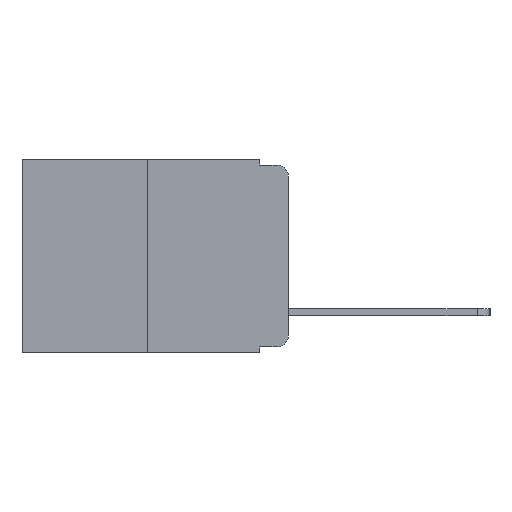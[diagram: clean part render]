
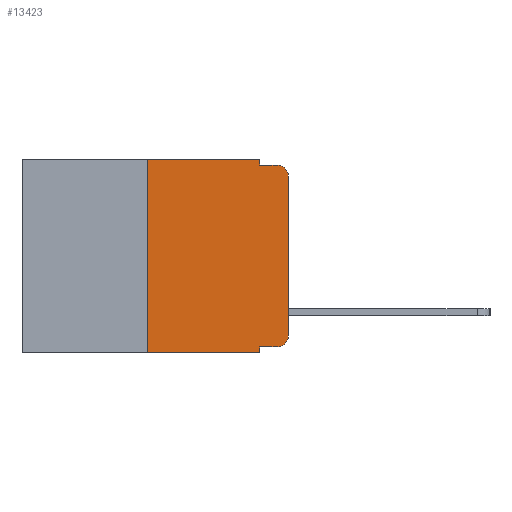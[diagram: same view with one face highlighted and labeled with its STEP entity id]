
A CAD part, left-side view. The second image highlights one B-rep face of the part: STEP entity #13423.
In plain terms, the highlighted planar face has unit normal (-1, 0, 0).
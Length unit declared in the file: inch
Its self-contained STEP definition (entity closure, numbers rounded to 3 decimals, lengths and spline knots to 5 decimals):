
#88 = AXIS2_PLACEMENT_3D ( 'NONE', #2605, #11744, #22862 ) ;
#1065 = CARTESIAN_POINT ( 'NONE',  ( 0., 0.051, 0. ) ) ;
#1620 = DIRECTION ( 'NONE',  ( 0., 0., 1. ) ) ;
#1627 = CARTESIAN_POINT ( 'NONE',  ( 0., 0.051, -0.01 ) ) ;
#1866 = EDGE_CURVE ( 'NONE', #9537, #21840, #20682, .T. ) ;
#1930 = VERTEX_POINT ( 'NONE', #1065 ) ;
#2000 = LINE ( 'NONE', #10922, #16400 ) ;
#2103 = LINE ( 'NONE', #11504, #17095 ) ;
#2592 = VECTOR ( 'NONE', #14992, 39.37008 ) ;
#2605 = CARTESIAN_POINT ( 'NONE',  ( 0., 0.02, -0.03 ) ) ;
#2713 = VERTEX_POINT ( 'NONE', #7784 ) ;
#3090 = LINE ( 'NONE', #24784, #12928 ) ;
#3095 = VECTOR ( 'NONE', #11310, 39.37008 ) ;
#3607 = VERTEX_POINT ( 'NONE', #5575 ) ;
#3814 = CARTESIAN_POINT ( 'NONE',  ( 0., 0.02, -0.333 ) ) ;
#4448 = CARTESIAN_POINT ( 'NONE',  ( 0., 0.051, 0. ) ) ;
#5096 = EDGE_CURVE ( 'NONE', #22543, #3607, #7813, .T. ) ;
#5575 = CARTESIAN_POINT ( 'NONE',  ( 0., 0.051, -0.343 ) ) ;
#5905 = ORIENTED_EDGE ( 'NONE', *, *, #12785, .T. ) ;
#6699 = EDGE_CURVE ( 'NONE', #22543, #2713, #17188, .T. ) ;
#6916 = CIRCLE ( 'NONE', #16382, 0.02 ) ;
#7174 = DIRECTION ( 'NONE',  ( 1., 0., 0. ) ) ;
#7784 = CARTESIAN_POINT ( 'NONE',  ( 0., 0.25, 0. ) ) ;
#7793 = VERTEX_POINT ( 'NONE', #20687 ) ;
#7813 = LINE ( 'NONE', #18756, #2592 ) ;
#7919 = ORIENTED_EDGE ( 'NONE', *, *, #17994, .F. ) ;
#8038 = VERTEX_POINT ( 'NONE', #13846 ) ;
#8069 = ORIENTED_EDGE ( 'NONE', *, *, #21421, .F. ) ;
#8320 = LINE ( 'NONE', #18988, #3095 ) ;
#8823 = CARTESIAN_POINT ( 'NONE',  ( 0., 0.02, -0.313 ) ) ;
#8953 = EDGE_CURVE ( 'NONE', #23219, #7793, #6916, .T. ) ;
#9537 = VERTEX_POINT ( 'NONE', #20189 ) ;
#10070 = EDGE_LOOP ( 'NONE', ( #12822, #24731, #18253, #24450, #7919, #15631, #20151, #8069, #5905, #21948 ) ) ;
#10779 = VECTOR ( 'NONE', #24455, 39.37008 ) ;
#10809 = DIRECTION ( 'NONE',  ( 0., 0., -1. ) ) ;
#10922 = CARTESIAN_POINT ( 'NONE',  ( 0., 0.473, 0. ) ) ;
#10969 = CARTESIAN_POINT ( 'NONE',  ( 0., 0.473, 0. ) ) ;
#11082 = CARTESIAN_POINT ( 'NONE',  ( 0., 0.051, -0.333 ) ) ;
#11161 = LINE ( 'NONE', #4448, #11768 ) ;
#11310 = DIRECTION ( 'NONE',  ( 0., 0., -1. ) ) ;
#11504 = CARTESIAN_POINT ( 'NONE',  ( 0., 0.051, -0.01 ) ) ;
#11744 = DIRECTION ( 'NONE',  ( -1., 0., 0. ) ) ;
#11768 = VECTOR ( 'NONE', #19919, 39.37008 ) ;
#12285 = CARTESIAN_POINT ( 'NONE',  ( 0., 0.25, 0. ) ) ;
#12785 = EDGE_CURVE ( 'NONE', #8038, #23219, #15350, .T. ) ;
#12822 = ORIENTED_EDGE ( 'NONE', *, *, #12909, .T. ) ;
#12905 = DIRECTION ( 'NONE',  ( 0., -1., 0. ) ) ;
#12909 = EDGE_CURVE ( 'NONE', #7793, #9537, #3090, .T. ) ;
#12928 = VECTOR ( 'NONE', #1620, 39.37008 ) ;
#13032 = PLANE ( 'NONE',  #21058 ) ;
#13423 = ADVANCED_FACE ( 'NONE', ( #20182 ), #13032, .F. ) ;
#13543 = CARTESIAN_POINT ( 'NONE',  ( 0., 0.02, -0.01 ) ) ;
#13710 = CARTESIAN_POINT ( 'NONE',  ( 0., 0.25, -0.343 ) ) ;
#13846 = CARTESIAN_POINT ( 'NONE',  ( 0., 0.051, -0.333 ) ) ;
#14992 = DIRECTION ( 'NONE',  ( 0., -1., 0. ) ) ;
#15202 = EDGE_CURVE ( 'NONE', #1930, #18199, #8320, .T. ) ;
#15350 = LINE ( 'NONE', #11082, #10779 ) ;
#15631 = ORIENTED_EDGE ( 'NONE', *, *, #6699, .F. ) ;
#16313 = EDGE_CURVE ( 'NONE', #18199, #21840, #2103, .T. ) ;
#16382 = AXIS2_PLACEMENT_3D ( 'NONE', #8823, #22262, #10809 ) ;
#16400 = VECTOR ( 'NONE', #12905, 39.37008 ) ;
#16587 = VECTOR ( 'NONE', #23712, 39.37008 ) ;
#17095 = VECTOR ( 'NONE', #22968, 39.37008 ) ;
#17188 = LINE ( 'NONE', #12285, #16587 ) ;
#17994 = EDGE_CURVE ( 'NONE', #2713, #1930, #2000, .T. ) ;
#18199 = VERTEX_POINT ( 'NONE', #1627 ) ;
#18253 = ORIENTED_EDGE ( 'NONE', *, *, #16313, .F. ) ;
#18756 = CARTESIAN_POINT ( 'NONE',  ( 0., 0.473, -0.343 ) ) ;
#18988 = CARTESIAN_POINT ( 'NONE',  ( 0., 0.051, 0. ) ) ;
#19919 = DIRECTION ( 'NONE',  ( 0., 0., -1. ) ) ;
#20151 = ORIENTED_EDGE ( 'NONE', *, *, #5096, .T. ) ;
#20182 = FACE_OUTER_BOUND ( 'NONE', #10070, .T. ) ;
#20189 = CARTESIAN_POINT ( 'NONE',  ( 0., 0., -0.03 ) ) ;
#20682 = CIRCLE ( 'NONE', #88, 0.02 ) ;
#20687 = CARTESIAN_POINT ( 'NONE',  ( 0., 0., -0.313 ) ) ;
#20703 = DIRECTION ( 'NONE',  ( 0., 0., -1. ) ) ;
#21058 = AXIS2_PLACEMENT_3D ( 'NONE', #10969, #7174, #20703 ) ;
#21421 = EDGE_CURVE ( 'NONE', #8038, #3607, #11161, .T. ) ;
#21840 = VERTEX_POINT ( 'NONE', #13543 ) ;
#21948 = ORIENTED_EDGE ( 'NONE', *, *, #8953, .T. ) ;
#22262 = DIRECTION ( 'NONE',  ( -1., 0., 0. ) ) ;
#22543 = VERTEX_POINT ( 'NONE', #13710 ) ;
#22862 = DIRECTION ( 'NONE',  ( 0., 0., -1. ) ) ;
#22968 = DIRECTION ( 'NONE',  ( 0., -1., 0. ) ) ;
#23219 = VERTEX_POINT ( 'NONE', #3814 ) ;
#23712 = DIRECTION ( 'NONE',  ( 0., 0., 1. ) ) ;
#24450 = ORIENTED_EDGE ( 'NONE', *, *, #15202, .F. ) ;
#24455 = DIRECTION ( 'NONE',  ( 0., -1., 0. ) ) ;
#24731 = ORIENTED_EDGE ( 'NONE', *, *, #1866, .T. ) ;
#24784 = CARTESIAN_POINT ( 'NONE',  ( 0., 0., 0. ) ) ;
